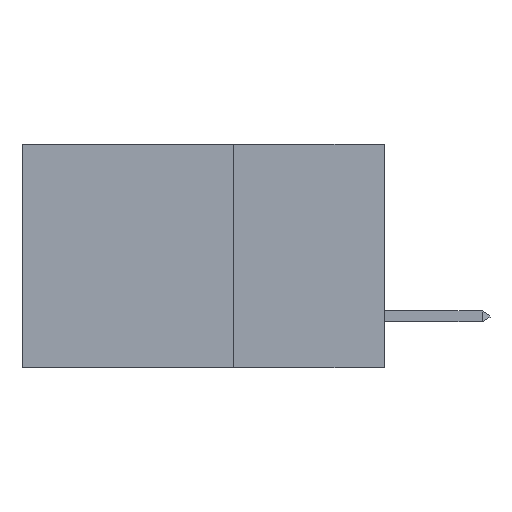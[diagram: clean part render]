
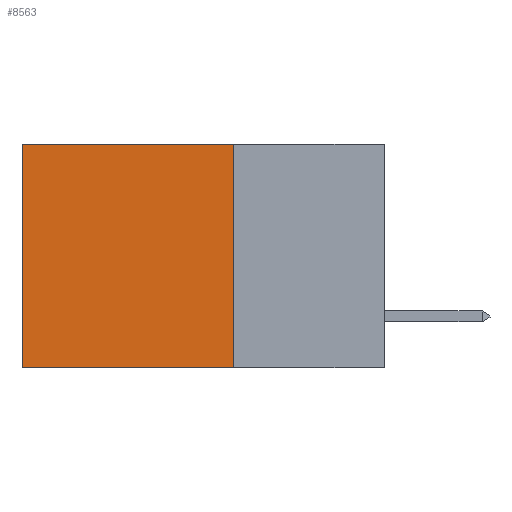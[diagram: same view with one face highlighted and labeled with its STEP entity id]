
A CAD part, left-side view. The second image highlights one B-rep face of the part: STEP entity #8563.
In plain terms, the highlighted planar face has unit normal (-1, 0, 0).
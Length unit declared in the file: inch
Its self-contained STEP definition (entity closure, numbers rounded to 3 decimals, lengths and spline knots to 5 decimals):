
#1545 = VECTOR ( 'NONE', #10208, 39.37008 ) ;
#1760 = LINE ( 'NONE', #15593, #8408 ) ;
#3037 = ORIENTED_EDGE ( 'NONE', *, *, #18122, .T. ) ;
#3680 = CARTESIAN_POINT ( 'NONE',  ( 0.2875, 0.25, 0. ) ) ;
#5813 = EDGE_CURVE ( 'NONE', #15917, #30956, #34625, .T. ) ;
#7225 = CARTESIAN_POINT ( 'NONE',  ( 0.2875, 0.25, -0.37 ) ) ;
#8149 = CARTESIAN_POINT ( 'NONE',  ( 0.2875, 0.6, 0. ) ) ;
#8408 = VECTOR ( 'NONE', #31289, 39.37008 ) ;
#8563 = ADVANCED_FACE ( 'NONE', ( #20319 ), #12020, .F. ) ;
#9077 = LINE ( 'NONE', #28637, #1545 ) ;
#10208 = DIRECTION ( 'NONE',  ( 0., 0., -1. ) ) ;
#11008 = EDGE_CURVE ( 'NONE', #30956, #11661, #1760, .T. ) ;
#11257 = EDGE_LOOP ( 'NONE', ( #29042, #22968, #24591, #3037 ) ) ;
#11661 = VERTEX_POINT ( 'NONE', #25985 ) ;
#12020 = PLANE ( 'NONE',  #24922 ) ;
#14023 = VERTEX_POINT ( 'NONE', #8149 ) ;
#14728 = DIRECTION ( 'NONE',  ( 0., 0., -1. ) ) ;
#15593 = CARTESIAN_POINT ( 'NONE',  ( 0.2875, 0.25, -0.37 ) ) ;
#15917 = VERTEX_POINT ( 'NONE', #18661 ) ;
#18122 = EDGE_CURVE ( 'NONE', #15917, #14023, #21363, .T. ) ;
#18202 = DIRECTION ( 'NONE',  ( 0., 0., -1. ) ) ;
#18661 = CARTESIAN_POINT ( 'NONE',  ( 0.2875, 0.25, 0. ) ) ;
#19696 = EDGE_CURVE ( 'NONE', #14023, #11661, #9077, .T. ) ;
#20319 = FACE_OUTER_BOUND ( 'NONE', #11257, .T. ) ;
#21363 = LINE ( 'NONE', #28933, #27479 ) ;
#22968 = ORIENTED_EDGE ( 'NONE', *, *, #11008, .F. ) ;
#24591 = ORIENTED_EDGE ( 'NONE', *, *, #5813, .F. ) ;
#24922 = AXIS2_PLACEMENT_3D ( 'NONE', #3680, #30454, #14728 ) ;
#25985 = CARTESIAN_POINT ( 'NONE',  ( 0.2875, 0.6, -0.37 ) ) ;
#27479 = VECTOR ( 'NONE', #34001, 39.37008 ) ;
#27782 = VECTOR ( 'NONE', #18202, 39.37008 ) ;
#28637 = CARTESIAN_POINT ( 'NONE',  ( 0.2875, 0.6, 0. ) ) ;
#28933 = CARTESIAN_POINT ( 'NONE',  ( 0.2875, 0.25, 0. ) ) ;
#29042 = ORIENTED_EDGE ( 'NONE', *, *, #19696, .T. ) ;
#30454 = DIRECTION ( 'NONE',  ( 1., 0., 0. ) ) ;
#30956 = VERTEX_POINT ( 'NONE', #7225 ) ;
#31289 = DIRECTION ( 'NONE',  ( 0., 1., 0. ) ) ;
#33820 = CARTESIAN_POINT ( 'NONE',  ( 0.2875, 0.25, 0. ) ) ;
#34001 = DIRECTION ( 'NONE',  ( 0., 1., 0. ) ) ;
#34625 = LINE ( 'NONE', #33820, #27782 ) ;
